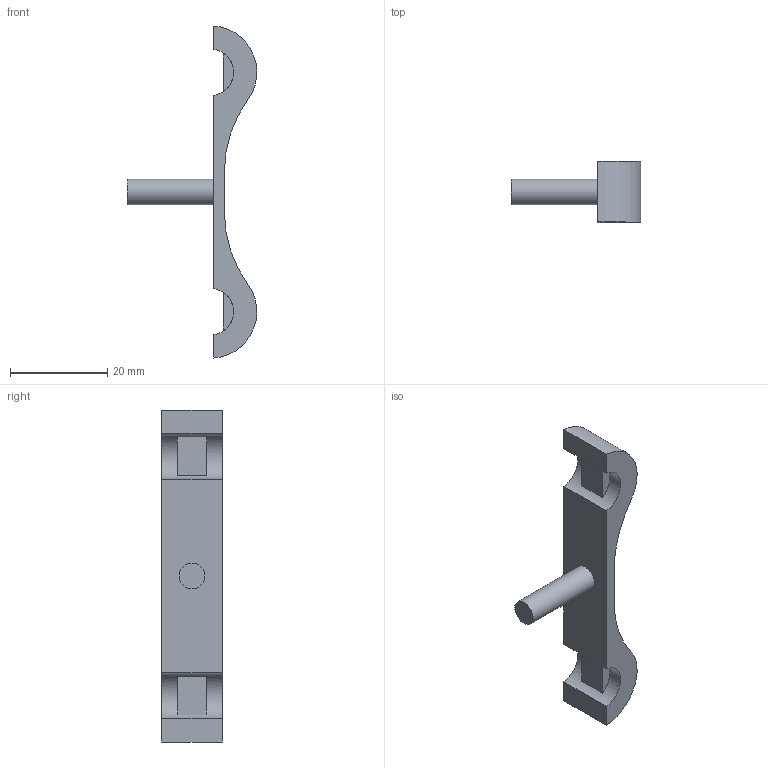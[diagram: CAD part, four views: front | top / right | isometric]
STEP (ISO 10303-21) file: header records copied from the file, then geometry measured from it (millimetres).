
FILE_DESCRIPTION (( 'STEP AP214' ), '1' );
FILE_NAME ('Arm Lock.STEP', '2014-02-12T12:47:23', ( 'elpi' ), ( '' ), 'SwSTEP 2.0', 'SolidWorks 2013', '' );
FILE_SCHEMA (( 'AUTOMOTIVE_DESIGN' ));
Length unit declared in the file: inch
Products named in the file (1): Arm Lock
Bounding box: 26.66 x 12.45 x 68.25 mm (x, y, z)
Volume: 4204.9 mm3; surface area: 2876.3 mm2
Topology: 1 solids, 1 shells, 20 faces, 46 edges, 31 vertices
Faces by surface type: plane 13, cylinder 7
Full cylindrical faces by diameter (mm): 5.334 x1
Entity records: 602 total; most frequent: DIRECTION 104, CARTESIAN_POINT 95, ORIENTED_EDGE 88, EDGE_CURVE 44, AXIS2_PLACEMENT_3D 39, VERTEX_POINT 30, VECTOR 26, LINE 26
